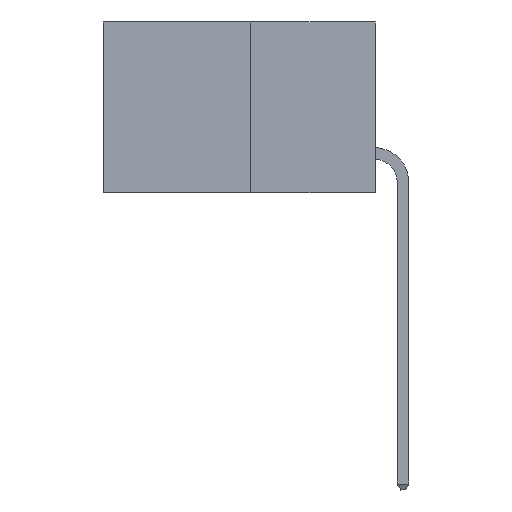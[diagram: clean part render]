
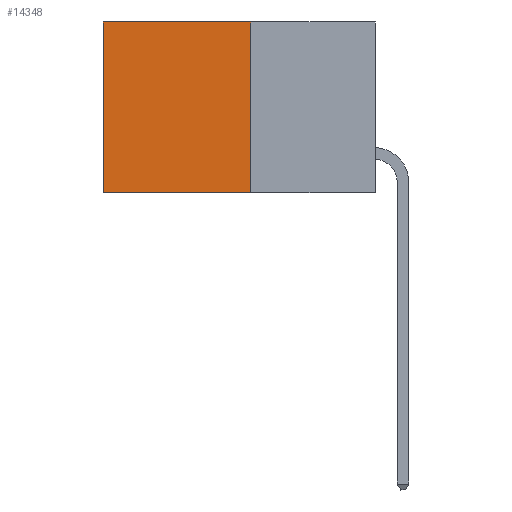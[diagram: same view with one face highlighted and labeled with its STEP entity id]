
A CAD part, left-side view. The second image highlights one B-rep face of the part: STEP entity #14348.
In plain terms, the highlighted planar face has unit normal (-1, 0, 0).
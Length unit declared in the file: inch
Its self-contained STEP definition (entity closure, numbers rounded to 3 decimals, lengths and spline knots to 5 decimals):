
#55 = DIRECTION ( 'NONE',  ( 1., 0., 0. ) ) ;
#146 = FACE_OUTER_BOUND ( 'NONE', #7798, .T. ) ;
#227 = VECTOR ( 'NONE', #10016, 39.37008 ) ;
#1355 = CARTESIAN_POINT ( 'NONE',  ( 0.277, 0.27, -0.37 ) ) ;
#2756 = ORIENTED_EDGE ( 'NONE', *, *, #15446, .F. ) ;
#3102 = LINE ( 'NONE', #7465, #13109 ) ;
#3105 = DIRECTION ( 'NONE',  ( 0., 0., -1. ) ) ;
#3922 = LINE ( 'NONE', #16468, #8199 ) ;
#4100 = LINE ( 'NONE', #1355, #227 ) ;
#4853 = CARTESIAN_POINT ( 'NONE',  ( 0.277, 0.27, -0.37 ) ) ;
#5335 = VERTEX_POINT ( 'NONE', #9358 ) ;
#5383 = CARTESIAN_POINT ( 'NONE',  ( 0.277, 0.27, -0.37 ) ) ;
#6412 = CARTESIAN_POINT ( 'NONE',  ( 0.277, 0.59, 0. ) ) ;
#6912 = LINE ( 'NONE', #5383, #17696 ) ;
#7465 = CARTESIAN_POINT ( 'NONE',  ( 0.277, 0.59, -0.37 ) ) ;
#7798 = EDGE_LOOP ( 'NONE', ( #9029, #2756, #14555, #11253 ) ) ;
#8032 = DIRECTION ( 'NONE',  ( 0., 1., 0. ) ) ;
#8077 = EDGE_CURVE ( 'NONE', #5335, #13292, #3922, .T. ) ;
#8199 = VECTOR ( 'NONE', #8032, 39.37008 ) ;
#8683 = PLANE ( 'NONE',  #16092 ) ;
#8875 = EDGE_CURVE ( 'NONE', #5335, #16336, #6912, .T. ) ;
#9029 = ORIENTED_EDGE ( 'NONE', *, *, #14440, .T. ) ;
#9358 = CARTESIAN_POINT ( 'NONE',  ( 0.277, 0.27, 0. ) ) ;
#10016 = DIRECTION ( 'NONE',  ( 0., 1., 0. ) ) ;
#10098 = DIRECTION ( 'NONE',  ( 0., 0., -1. ) ) ;
#11253 = ORIENTED_EDGE ( 'NONE', *, *, #8077, .T. ) ;
#12965 = CARTESIAN_POINT ( 'NONE',  ( 0.277, 0.59, -0.37 ) ) ;
#13109 = VECTOR ( 'NONE', #3105, 39.37008 ) ;
#13292 = VERTEX_POINT ( 'NONE', #6412 ) ;
#14348 = ADVANCED_FACE ( 'NONE', ( #146 ), #8683, .F. ) ;
#14440 = EDGE_CURVE ( 'NONE', #13292, #15040, #3102, .T. ) ;
#14555 = ORIENTED_EDGE ( 'NONE', *, *, #8875, .F. ) ;
#15040 = VERTEX_POINT ( 'NONE', #12965 ) ;
#15446 = EDGE_CURVE ( 'NONE', #16336, #15040, #4100, .T. ) ;
#15713 = CARTESIAN_POINT ( 'NONE',  ( 0.277, 0.27, -0.37 ) ) ;
#16092 = AXIS2_PLACEMENT_3D ( 'NONE', #15713, #55, #10098 ) ;
#16336 = VERTEX_POINT ( 'NONE', #4853 ) ;
#16468 = CARTESIAN_POINT ( 'NONE',  ( 0.277, 0.27, 0. ) ) ;
#16679 = DIRECTION ( 'NONE',  ( 0., 0., -1. ) ) ;
#17696 = VECTOR ( 'NONE', #16679, 39.37008 ) ;
